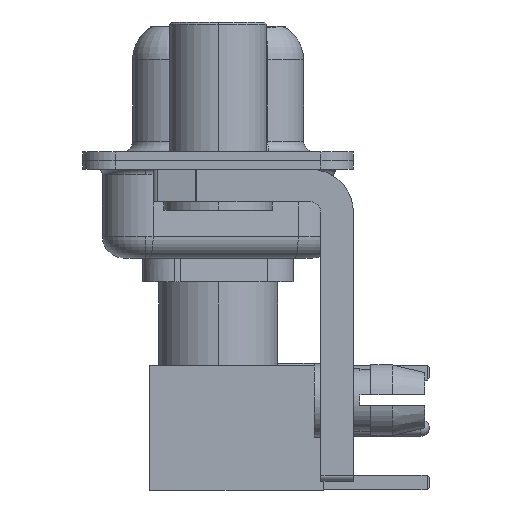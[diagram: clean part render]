
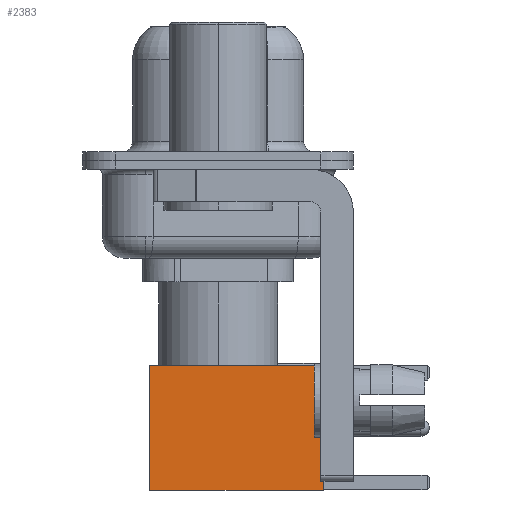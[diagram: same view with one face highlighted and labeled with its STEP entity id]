
A CAD part, left-side view. The second image highlights one B-rep face of the part: STEP entity #2383.
In plain terms, the highlighted face is planar.
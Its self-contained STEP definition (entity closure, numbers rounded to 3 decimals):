
#484 = DIRECTION ( 'NONE',  ( 0., 0., 1. ) ) ;
#1773 = VECTOR ( 'NONE', #20797, 1000. ) ;
#2051 = EDGE_CURVE ( 'NONE', #12413, #8134, #8825, .T. ) ;
#2383 = ADVANCED_FACE ( 'NONE', ( #2885 ), #27077, .T. ) ;
#2745 = ORIENTED_EDGE ( 'NONE', *, *, #29622, .T. ) ;
#2885 = FACE_OUTER_BOUND ( 'NONE', #31142, .T. ) ;
#2903 = CARTESIAN_POINT ( 'NONE',  ( -2.875, 2.875, 0. ) ) ;
#3559 = CARTESIAN_POINT ( 'NONE',  ( 0., 2.875, 0. ) ) ;
#3750 = ORIENTED_EDGE ( 'NONE', *, *, #2051, .F. ) ;
#5849 = EDGE_CURVE ( 'NONE', #13739, #26244, #30284, .T. ) ;
#6425 = CARTESIAN_POINT ( 'NONE',  ( 0., 2.875, 8. ) ) ;
#8134 = VERTEX_POINT ( 'NONE', #17715 ) ;
#8137 = CARTESIAN_POINT ( 'NONE',  ( 2.875, 2.875, 0. ) ) ;
#8825 = LINE ( 'NONE', #6425, #24179 ) ;
#8880 = EDGE_CURVE ( 'NONE', #8134, #26244, #19899, .T. ) ;
#9210 = ORIENTED_EDGE ( 'NONE', *, *, #5849, .T. ) ;
#12413 = VERTEX_POINT ( 'NONE', #13076 ) ;
#12660 = CARTESIAN_POINT ( 'NONE',  ( 2.875, 2.875, 0. ) ) ;
#13076 = CARTESIAN_POINT ( 'NONE',  ( 2.875, 2.875, 8. ) ) ;
#13739 = VERTEX_POINT ( 'NONE', #19290 ) ;
#14339 = VECTOR ( 'NONE', #20211, 1000. ) ;
#16363 = DIRECTION ( 'NONE',  ( -1., 0., 0. ) ) ;
#16833 = DIRECTION ( 'NONE',  ( -1., 0., 0. ) ) ;
#17715 = CARTESIAN_POINT ( 'NONE',  ( -2.875, 2.875, 8. ) ) ;
#17978 = VECTOR ( 'NONE', #16363, 1000. ) ;
#19290 = CARTESIAN_POINT ( 'NONE',  ( 2.875, 2.875, 0. ) ) ;
#19599 = AXIS2_PLACEMENT_3D ( 'NONE', #12660, #22431, #484 ) ;
#19899 = LINE ( 'NONE', #2903, #14339 ) ;
#20211 = DIRECTION ( 'NONE',  ( 0., 0., -1. ) ) ;
#20797 = DIRECTION ( 'NONE',  ( 0., 0., -1. ) ) ;
#22431 = DIRECTION ( 'NONE',  ( 0., 1., 0. ) ) ;
#22569 = LINE ( 'NONE', #8137, #1773 ) ;
#24179 = VECTOR ( 'NONE', #16833, 1000. ) ;
#26244 = VERTEX_POINT ( 'NONE', #29889 ) ;
#27077 = PLANE ( 'NONE',  #19599 ) ;
#28398 = ORIENTED_EDGE ( 'NONE', *, *, #8880, .F. ) ;
#29622 = EDGE_CURVE ( 'NONE', #12413, #13739, #22569, .T. ) ;
#29889 = CARTESIAN_POINT ( 'NONE',  ( -2.875, 2.875, 0. ) ) ;
#30284 = LINE ( 'NONE', #3559, #17978 ) ;
#31142 = EDGE_LOOP ( 'NONE', ( #2745, #9210, #28398, #3750 ) ) ;
